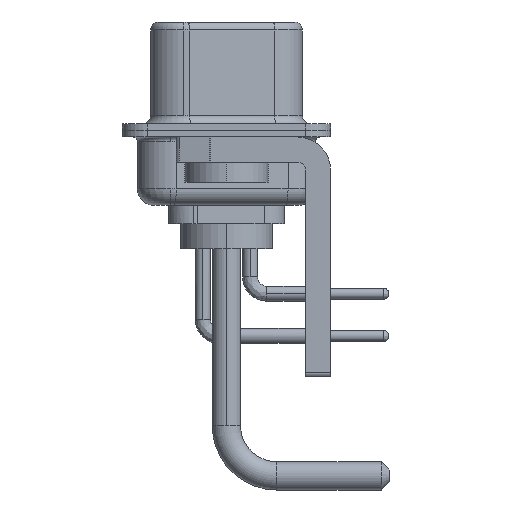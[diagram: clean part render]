
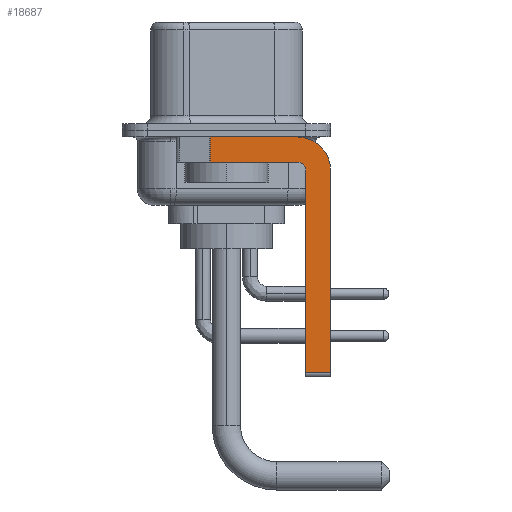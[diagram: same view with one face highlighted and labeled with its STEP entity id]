
A CAD part, left-side view. The second image highlights one B-rep face of the part: STEP entity #18687.
In plain terms, the highlighted planar face has unit normal (-1, 0, 0).
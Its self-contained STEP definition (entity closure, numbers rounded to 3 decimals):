
#88 = ORIENTED_EDGE ( 'NONE', *, *, #183, .F. ) ;
#100 = VERTEX_POINT ( 'NONE', #10730 ) ;
#183 = EDGE_CURVE ( 'NONE', #20151, #100, #21759, .T. ) ;
#381 = DIRECTION ( 'NONE',  ( 0., 0., -1. ) ) ;
#429 = VERTEX_POINT ( 'NONE', #14916 ) ;
#444 = ORIENTED_EDGE ( 'NONE', *, *, #19532, .F. ) ;
#553 = EDGE_CURVE ( 'NONE', #100, #11498, #17576, .T. ) ;
#1880 = CARTESIAN_POINT ( 'NONE',  ( -2.9, -6.25, -14.55 ) ) ;
#2400 = CARTESIAN_POINT ( 'NONE',  ( -2.9, -4.25, -2.4 ) ) ;
#2979 = VERTEX_POINT ( 'NONE', #14332 ) ;
#3051 = VECTOR ( 'NONE', #22965, 1000. ) ;
#3752 = DIRECTION ( 'NONE',  ( 0., 0., -1. ) ) ;
#4145 = AXIS2_PLACEMENT_3D ( 'NONE', #2400, #18795, #381 ) ;
#4207 = DIRECTION ( 'NONE',  ( -1., 0., 0. ) ) ;
#4656 = PLANE ( 'NONE',  #26562 ) ;
#6745 = VERTEX_POINT ( 'NONE', #8698 ) ;
#6746 = DIRECTION ( 'NONE',  ( 0., 0., 1. ) ) ;
#7171 = ORIENTED_EDGE ( 'NONE', *, *, #553, .F. ) ;
#8592 = ORIENTED_EDGE ( 'NONE', *, *, #20768, .F. ) ;
#8698 = CARTESIAN_POINT ( 'NONE',  ( -2.9, -4.25, -1.9 ) ) ;
#9143 = CARTESIAN_POINT ( 'NONE',  ( -2.9, -4.75, -14.8 ) ) ;
#9194 = AXIS2_PLACEMENT_3D ( 'NONE', #18166, #4207, #18698 ) ;
#9574 = EDGE_CURVE ( 'NONE', #429, #6745, #20784, .T. ) ;
#10730 = CARTESIAN_POINT ( 'NONE',  ( -2.9, -6.25, -2.4 ) ) ;
#11498 = VERTEX_POINT ( 'NONE', #1880 ) ;
#11787 = EDGE_LOOP ( 'NONE', ( #19403, #20625, #8592, #25317, #444, #13526, #7171, #88 ) ) ;
#11984 = VERTEX_POINT ( 'NONE', #14047 ) ;
#12311 = CARTESIAN_POINT ( 'NONE',  ( -2.9, -4.25, -0.4 ) ) ;
#12436 = VECTOR ( 'NONE', #6746, 1000. ) ;
#12578 = VECTOR ( 'NONE', #17831, 1000. ) ;
#13520 = VERTEX_POINT ( 'NONE', #15084 ) ;
#13526 = ORIENTED_EDGE ( 'NONE', *, *, #22039, .T. ) ;
#14047 = CARTESIAN_POINT ( 'NONE',  ( -2.9, 0.978, -1.9 ) ) ;
#14332 = CARTESIAN_POINT ( 'NONE',  ( -2.9, 0.978, -0.4 ) ) ;
#14696 = VECTOR ( 'NONE', #26133, 1000. ) ;
#14749 = CARTESIAN_POINT ( 'NONE',  ( -2.9, -4.25, -1.9 ) ) ;
#14863 = FACE_OUTER_BOUND ( 'NONE', #11787, .T. ) ;
#14916 = CARTESIAN_POINT ( 'NONE',  ( -2.9, -4.75, -2.4 ) ) ;
#15084 = CARTESIAN_POINT ( 'NONE',  ( -2.9, -4.75, -14.55 ) ) ;
#15961 = DIRECTION ( 'NONE',  ( 0., 0., -1. ) ) ;
#16139 = CARTESIAN_POINT ( 'NONE',  ( -2.9, 3., -0.4 ) ) ;
#16280 = LINE ( 'NONE', #16139, #19821 ) ;
#16319 = LINE ( 'NONE', #17926, #14696 ) ;
#16814 = LINE ( 'NONE', #9143, #12436 ) ;
#17576 = LINE ( 'NONE', #19844, #12578 ) ;
#17831 = DIRECTION ( 'NONE',  ( 0., 0., -1. ) ) ;
#17926 = CARTESIAN_POINT ( 'NONE',  ( -2.9, -4.25, -14.55 ) ) ;
#18166 = CARTESIAN_POINT ( 'NONE',  ( -2.9, -4.25, -2.4 ) ) ;
#18678 = DIRECTION ( 'NONE',  ( 0., -1., 0. ) ) ;
#18687 = ADVANCED_FACE ( 'NONE', ( #14863 ), #4656, .F. ) ;
#18698 = DIRECTION ( 'NONE',  ( 0., 0., 1. ) ) ;
#18795 = DIRECTION ( 'NONE',  ( 1., 0., 0. ) ) ;
#19403 = ORIENTED_EDGE ( 'NONE', *, *, #21548, .F. ) ;
#19532 = EDGE_CURVE ( 'NONE', #13520, #429, #16814, .T. ) ;
#19821 = VECTOR ( 'NONE', #18678, 1000. ) ;
#19844 = CARTESIAN_POINT ( 'NONE',  ( -2.9, -6.25, -2.4 ) ) ;
#20140 = LINE ( 'NONE', #24312, #23249 ) ;
#20151 = VERTEX_POINT ( 'NONE', #12311 ) ;
#20562 = EDGE_CURVE ( 'NONE', #2979, #11984, #20140, .T. ) ;
#20625 = ORIENTED_EDGE ( 'NONE', *, *, #20562, .T. ) ;
#20643 = CARTESIAN_POINT ( 'NONE',  ( -2.9, -4.25, -2.4 ) ) ;
#20768 = EDGE_CURVE ( 'NONE', #6745, #11984, #25252, .T. ) ;
#20784 = CIRCLE ( 'NONE', #9194, 0.5 ) ;
#21548 = EDGE_CURVE ( 'NONE', #2979, #20151, #16280, .T. ) ;
#21759 = CIRCLE ( 'NONE', #4145, 2. ) ;
#22039 = EDGE_CURVE ( 'NONE', #13520, #11498, #16319, .T. ) ;
#22169 = DIRECTION ( 'NONE',  ( 1., 0., 0. ) ) ;
#22965 = DIRECTION ( 'NONE',  ( 0., 1., 0. ) ) ;
#23249 = VECTOR ( 'NONE', #15961, 1000. ) ;
#24312 = CARTESIAN_POINT ( 'NONE',  ( -2.9, 0.978, -1.9 ) ) ;
#25252 = LINE ( 'NONE', #14749, #3051 ) ;
#25317 = ORIENTED_EDGE ( 'NONE', *, *, #9574, .F. ) ;
#26133 = DIRECTION ( 'NONE',  ( 0., -1., 0. ) ) ;
#26562 = AXIS2_PLACEMENT_3D ( 'NONE', #20643, #22169, #3752 ) ;
